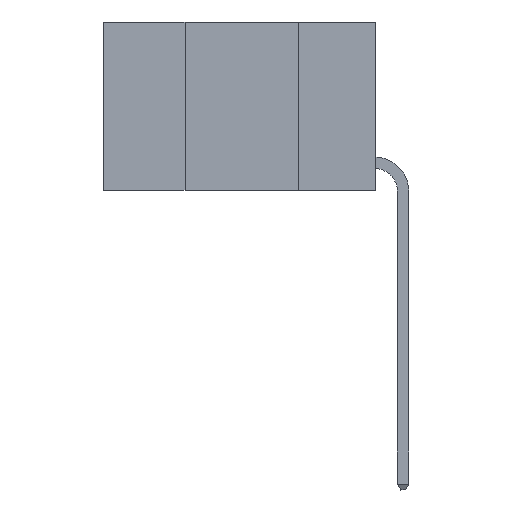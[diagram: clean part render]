
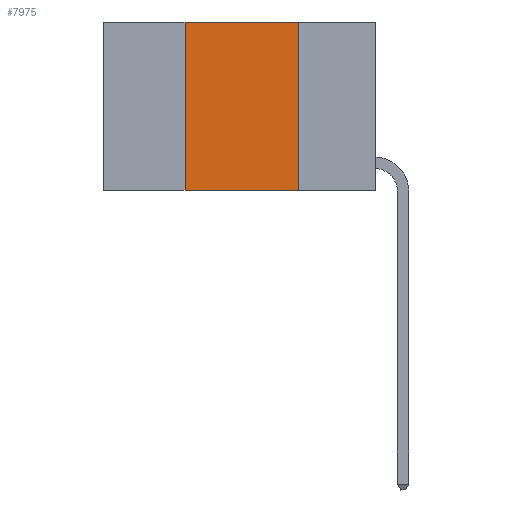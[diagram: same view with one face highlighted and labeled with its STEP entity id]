
A CAD part, left-side view. The second image highlights one B-rep face of the part: STEP entity #7975.
In plain terms, the highlighted planar face has unit normal (-1, 0, 0).
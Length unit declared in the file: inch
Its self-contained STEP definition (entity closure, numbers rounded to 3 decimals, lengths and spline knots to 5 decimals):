
#23 = VERTEX_POINT ( 'NONE', #7710 ) ;
#70 = AXIS2_PLACEMENT_3D ( 'NONE', #6469, #9687, #2855 ) ;
#122 = VECTOR ( 'NONE', #10307, 39.37008 ) ;
#1627 = DIRECTION ( 'NONE',  ( 0., -1., 0. ) ) ;
#2225 = EDGE_CURVE ( 'NONE', #23, #3956, #8838, .T. ) ;
#2855 = DIRECTION ( 'NONE',  ( 0., 0., -1. ) ) ;
#2936 = ORIENTED_EDGE ( 'NONE', *, *, #2225, .F. ) ;
#3363 = VERTEX_POINT ( 'NONE', #12593 ) ;
#3956 = VERTEX_POINT ( 'NONE', #7133 ) ;
#4413 = ORIENTED_EDGE ( 'NONE', *, *, #11942, .F. ) ;
#4600 = VECTOR ( 'NONE', #8297, 39.37008 ) ;
#5053 = ORIENTED_EDGE ( 'NONE', *, *, #9858, .T. ) ;
#5064 = DIRECTION ( 'NONE',  ( 0., 0., -1. ) ) ;
#6002 = EDGE_CURVE ( 'NONE', #3363, #23, #9797, .T. ) ;
#6200 = CARTESIAN_POINT ( 'NONE',  ( 0., 0.17, 0. ) ) ;
#6469 = CARTESIAN_POINT ( 'NONE',  ( 0., 0.6, 0. ) ) ;
#7133 = CARTESIAN_POINT ( 'NONE',  ( 0., 0.17, 0. ) ) ;
#7429 = FACE_OUTER_BOUND ( 'NONE', #9342, .T. ) ;
#7710 = CARTESIAN_POINT ( 'NONE',  ( 0., 0.42, 0. ) ) ;
#7961 = VERTEX_POINT ( 'NONE', #8669 ) ;
#7975 = ADVANCED_FACE ( 'NONE', ( #7429 ), #8721, .F. ) ;
#8297 = DIRECTION ( 'NONE',  ( 0., 0., 1. ) ) ;
#8669 = CARTESIAN_POINT ( 'NONE',  ( 0., 0.17, -0.37 ) ) ;
#8721 = PLANE ( 'NONE',  #70 ) ;
#8838 = LINE ( 'NONE', #13405, #122 ) ;
#9015 = VECTOR ( 'NONE', #5064, 39.37008 ) ;
#9342 = EDGE_LOOP ( 'NONE', ( #4413, #2936, #10873, #5053 ) ) ;
#9687 = DIRECTION ( 'NONE',  ( 1., 0., 0. ) ) ;
#9797 = LINE ( 'NONE', #13131, #4600 ) ;
#9858 = EDGE_CURVE ( 'NONE', #3363, #7961, #10742, .T. ) ;
#10307 = DIRECTION ( 'NONE',  ( 0., -1., 0. ) ) ;
#10742 = LINE ( 'NONE', #12612, #12985 ) ;
#10873 = ORIENTED_EDGE ( 'NONE', *, *, #6002, .F. ) ;
#11608 = LINE ( 'NONE', #6200, #9015 ) ;
#11942 = EDGE_CURVE ( 'NONE', #3956, #7961, #11608, .T. ) ;
#12593 = CARTESIAN_POINT ( 'NONE',  ( 0., 0.42, -0.37 ) ) ;
#12612 = CARTESIAN_POINT ( 'NONE',  ( 0., 0.6, -0.37 ) ) ;
#12985 = VECTOR ( 'NONE', #1627, 39.37008 ) ;
#13131 = CARTESIAN_POINT ( 'NONE',  ( 0., 0.42, 0. ) ) ;
#13405 = CARTESIAN_POINT ( 'NONE',  ( 0., 0.6, 0. ) ) ;
